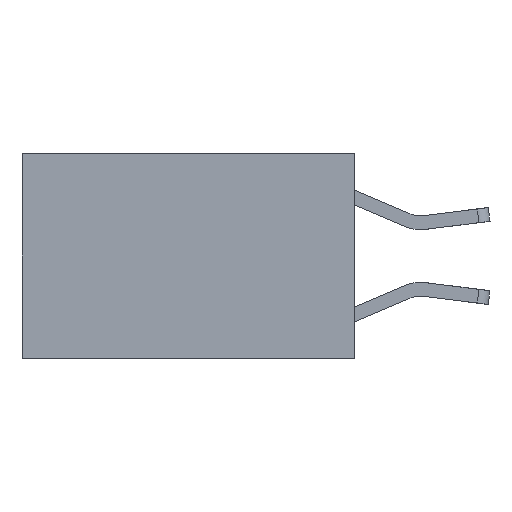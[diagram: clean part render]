
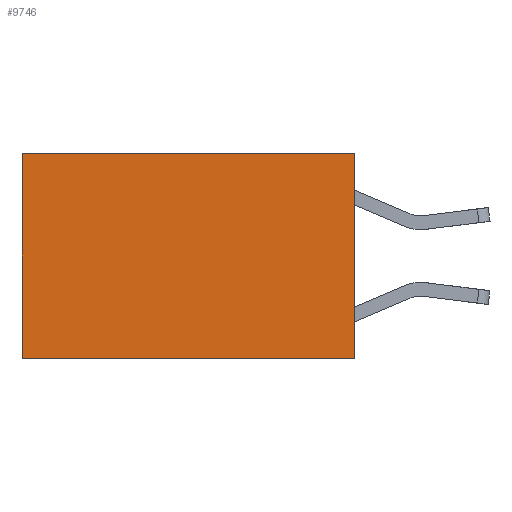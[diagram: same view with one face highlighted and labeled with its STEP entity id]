
A CAD part, left-side view. The second image highlights one B-rep face of the part: STEP entity #9746.
In plain terms, the highlighted planar face has unit normal (-1, 0, 0).
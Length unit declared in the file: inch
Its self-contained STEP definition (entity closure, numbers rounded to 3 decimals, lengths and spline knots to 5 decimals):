
#214 = CARTESIAN_POINT ( 'NONE',  ( 0.2625, 0.6, 0. ) ) ;
#260 = DIRECTION ( 'NONE',  ( 0., 0., -1. ) ) ;
#378 = LINE ( 'NONE', #10324, #2080 ) ;
#539 = CARTESIAN_POINT ( 'NONE',  ( 0.2625, 0., 0. ) ) ;
#1120 = ORIENTED_EDGE ( 'NONE', *, *, #3646, .F. ) ;
#1368 = DIRECTION ( 'NONE',  ( 0., 0., -1. ) ) ;
#1522 = DIRECTION ( 'NONE',  ( 0., 1., 0. ) ) ;
#1712 = LINE ( 'NONE', #4097, #7943 ) ;
#1953 = CARTESIAN_POINT ( 'NONE',  ( 0.2625, 0., 0. ) ) ;
#2080 = VECTOR ( 'NONE', #9491, 39.37008 ) ;
#2432 = CARTESIAN_POINT ( 'NONE',  ( 0.2625, 0., 0. ) ) ;
#2456 = VERTEX_POINT ( 'NONE', #7550 ) ;
#2750 = AXIS2_PLACEMENT_3D ( 'NONE', #539, #6277, #1368 ) ;
#2812 = ORIENTED_EDGE ( 'NONE', *, *, #5201, .T. ) ;
#3511 = EDGE_LOOP ( 'NONE', ( #6915, #9752, #1120, #2812 ) ) ;
#3646 = EDGE_CURVE ( 'NONE', #2456, #7635, #7400, .T. ) ;
#3827 = CARTESIAN_POINT ( 'NONE',  ( 0.2625, 0.6, -0.37 ) ) ;
#4097 = CARTESIAN_POINT ( 'NONE',  ( 0.2625, 0.6, 0. ) ) ;
#5010 = VECTOR ( 'NONE', #260, 39.37008 ) ;
#5170 = CARTESIAN_POINT ( 'NONE',  ( 0.2625, 0., -0.37 ) ) ;
#5201 = EDGE_CURVE ( 'NONE', #2456, #8142, #9157, .T. ) ;
#6277 = DIRECTION ( 'NONE',  ( 1., 0., 0. ) ) ;
#6502 = DIRECTION ( 'NONE',  ( 0., 0., -1. ) ) ;
#6915 = ORIENTED_EDGE ( 'NONE', *, *, #8683, .T. ) ;
#7042 = VECTOR ( 'NONE', #1522, 39.37008 ) ;
#7400 = LINE ( 'NONE', #1953, #5010 ) ;
#7550 = CARTESIAN_POINT ( 'NONE',  ( 0.2625, 0., 0. ) ) ;
#7635 = VERTEX_POINT ( 'NONE', #5170 ) ;
#7943 = VECTOR ( 'NONE', #6502, 39.37008 ) ;
#8142 = VERTEX_POINT ( 'NONE', #214 ) ;
#8555 = FACE_OUTER_BOUND ( 'NONE', #3511, .T. ) ;
#8683 = EDGE_CURVE ( 'NONE', #8142, #9735, #1712, .T. ) ;
#9157 = LINE ( 'NONE', #2432, #7042 ) ;
#9459 = PLANE ( 'NONE',  #2750 ) ;
#9491 = DIRECTION ( 'NONE',  ( 0., 1., 0. ) ) ;
#9735 = VERTEX_POINT ( 'NONE', #3827 ) ;
#9746 = ADVANCED_FACE ( 'NONE', ( #8555 ), #9459, .F. ) ;
#9752 = ORIENTED_EDGE ( 'NONE', *, *, #10392, .F. ) ;
#10324 = CARTESIAN_POINT ( 'NONE',  ( 0.2625, 0., -0.37 ) ) ;
#10392 = EDGE_CURVE ( 'NONE', #7635, #9735, #378, .T. ) ;
